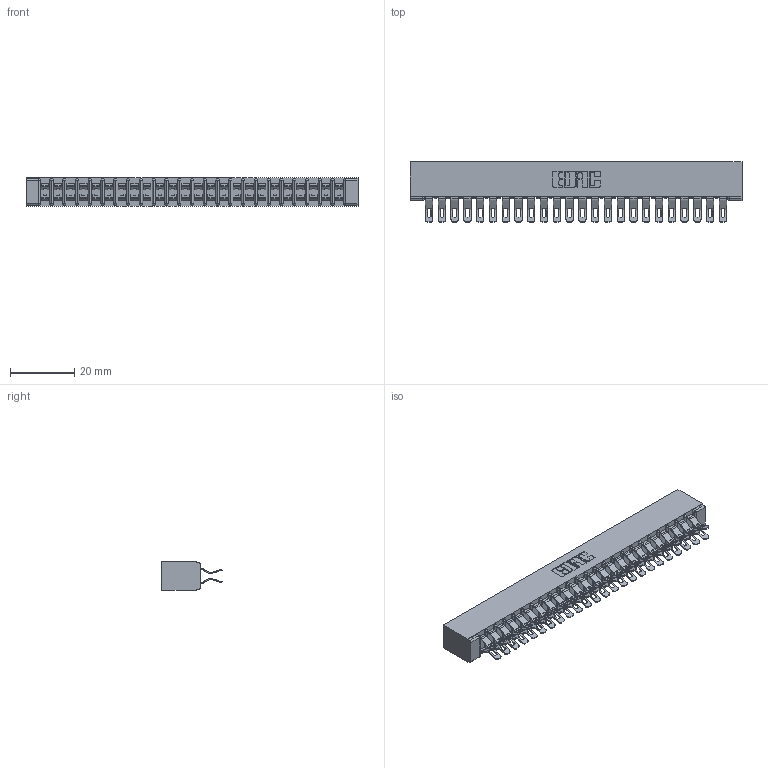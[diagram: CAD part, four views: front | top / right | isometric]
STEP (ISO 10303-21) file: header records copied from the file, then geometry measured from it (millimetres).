
FILE_DESCRIPTION (( 'STEP AP203' ), '1' );
FILE_NAME ('357-048-455-201.STEP', '2020-10-04T04:18:17', ( '' ), ( '' ), 'SwSTEP 2.0', 'SolidWorks 2020', '' );
FILE_SCHEMA (( 'CONFIG_CONTROL_DESIGN' ));
Length unit declared in the file: inch
Products named in the file (3): 307-290-001_555; 307 Part_No Mounting Lugs; 357-048-455-201
Assembly tree (49 placements, depth 2):
  357-048-455-201
    307 Part_No Mounting Lugs
    307-290-001_555  x48
Bounding box: 102.97 x 18.75 x 8.71 mm (x, y, z)
Volume: 7111.3 mm3; surface area: 13925.2 mm2
Topology: 49 solids, 49 shells, 3063 faces, 8987 edges, 5858 vertices
Faces by surface type: plane 1698, cylinder 1315, sphere 50
Entity records: 23821 total; most frequent: CARTESIAN_POINT 3904, ORIENTED_EDGE 3868, DIRECTION 3838, EDGE_CURVE 1934, LINE 1466, VECTOR 1466, VERTEX_POINT 1252, AXIS2_PLACEMENT_3D 1186
